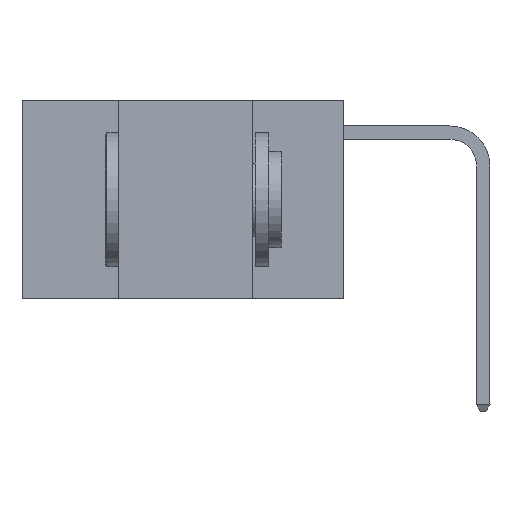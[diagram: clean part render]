
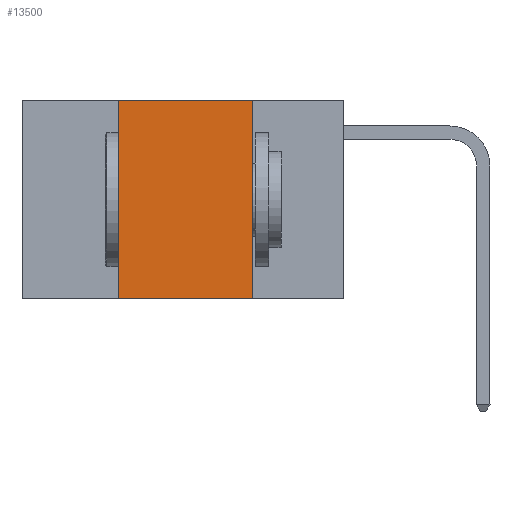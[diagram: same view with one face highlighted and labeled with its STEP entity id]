
A CAD part, left-side view. The second image highlights one B-rep face of the part: STEP entity #13500.
In plain terms, the highlighted planar face has unit normal (-1, 0, 0).
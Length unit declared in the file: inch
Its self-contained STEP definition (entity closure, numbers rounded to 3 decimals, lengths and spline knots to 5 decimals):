
#219 = DIRECTION ( 'NONE',  ( 0., 0., -1. ) ) ;
#363 = CARTESIAN_POINT ( 'NONE',  ( 0., 0.42, 0. ) ) ;
#389 = CARTESIAN_POINT ( 'NONE',  ( 0., 0.42, 0. ) ) ;
#1212 = PLANE ( 'NONE',  #4986 ) ;
#1521 = DIRECTION ( 'NONE',  ( 0., 0., 1. ) ) ;
#2260 = VERTEX_POINT ( 'NONE', #13036 ) ;
#2493 = CARTESIAN_POINT ( 'NONE',  ( 0., 0.17, 0. ) ) ;
#2713 = CARTESIAN_POINT ( 'NONE',  ( 0., 0.17, 0. ) ) ;
#3073 = VERTEX_POINT ( 'NONE', #7908 ) ;
#3416 = ORIENTED_EDGE ( 'NONE', *, *, #9624, .F. ) ;
#3525 = ORIENTED_EDGE ( 'NONE', *, *, #6032, .F. ) ;
#3583 = ORIENTED_EDGE ( 'NONE', *, *, #8946, .F. ) ;
#3611 = ORIENTED_EDGE ( 'NONE', *, *, #6844, .T. ) ;
#3815 = DIRECTION ( 'NONE',  ( 0., 0., -1. ) ) ;
#4195 = LINE ( 'NONE', #2713, #9595 ) ;
#4211 = EDGE_LOOP ( 'NONE', ( #3416, #3525, #3583, #3611 ) ) ;
#4986 = AXIS2_PLACEMENT_3D ( 'NONE', #13027, #6878, #219 ) ;
#5090 = VECTOR ( 'NONE', #5931, 39.37008 ) ;
#5270 = LINE ( 'NONE', #6280, #5090 ) ;
#5712 = VERTEX_POINT ( 'NONE', #2493 ) ;
#5931 = DIRECTION ( 'NONE',  ( 0., -1., 0. ) ) ;
#6032 = EDGE_CURVE ( 'NONE', #11181, #5712, #7510, .T. ) ;
#6280 = CARTESIAN_POINT ( 'NONE',  ( 0., 0.6, -0.37 ) ) ;
#6844 = EDGE_CURVE ( 'NONE', #2260, #3073, #5270, .T. ) ;
#6878 = DIRECTION ( 'NONE',  ( 1., 0., 0. ) ) ;
#7451 = VECTOR ( 'NONE', #12446, 39.37008 ) ;
#7510 = LINE ( 'NONE', #12437, #7451 ) ;
#7908 = CARTESIAN_POINT ( 'NONE',  ( 0., 0.17, -0.37 ) ) ;
#8328 = LINE ( 'NONE', #389, #10775 ) ;
#8946 = EDGE_CURVE ( 'NONE', #2260, #11181, #8328, .T. ) ;
#9595 = VECTOR ( 'NONE', #3815, 39.37008 ) ;
#9624 = EDGE_CURVE ( 'NONE', #5712, #3073, #4195, .T. ) ;
#10775 = VECTOR ( 'NONE', #1521, 39.37008 ) ;
#11181 = VERTEX_POINT ( 'NONE', #363 ) ;
#12437 = CARTESIAN_POINT ( 'NONE',  ( 0., 0.6, 0. ) ) ;
#12446 = DIRECTION ( 'NONE',  ( 0., -1., 0. ) ) ;
#12693 = FACE_OUTER_BOUND ( 'NONE', #4211, .T. ) ;
#13027 = CARTESIAN_POINT ( 'NONE',  ( 0., 0.6, 0. ) ) ;
#13036 = CARTESIAN_POINT ( 'NONE',  ( 0., 0.42, -0.37 ) ) ;
#13500 = ADVANCED_FACE ( 'NONE', ( #12693 ), #1212, .F. ) ;
